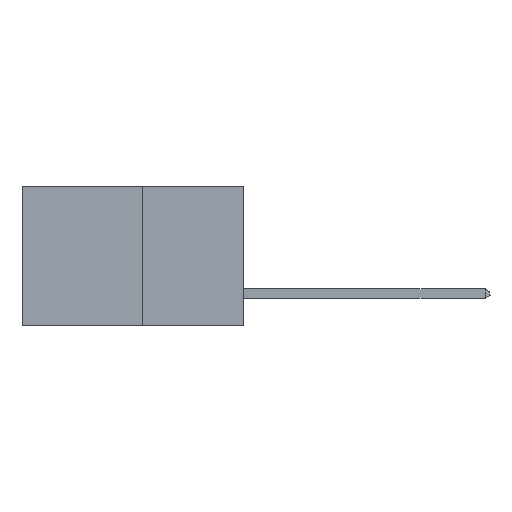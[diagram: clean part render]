
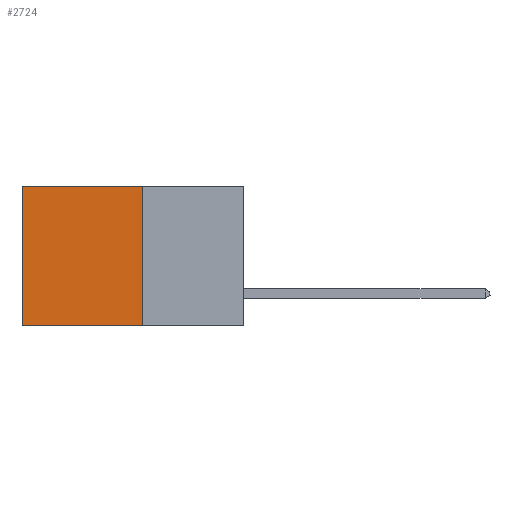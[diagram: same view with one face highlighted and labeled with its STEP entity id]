
A CAD part, left-side view. The second image highlights one B-rep face of the part: STEP entity #2724.
In plain terms, the highlighted planar face has unit normal (-1, 0, 0).
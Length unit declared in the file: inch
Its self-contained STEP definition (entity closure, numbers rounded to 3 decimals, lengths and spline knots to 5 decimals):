
#101 = AXIS2_PLACEMENT_3D ( 'NONE', #4078, #1665, #5378 ) ;
#337 = DIRECTION ( 'NONE',  ( 0., 1., 0. ) ) ;
#406 = DIRECTION ( 'NONE',  ( 0., 0., -1. ) ) ;
#720 = VERTEX_POINT ( 'NONE', #4737 ) ;
#1048 = CARTESIAN_POINT ( 'NONE',  ( 0.277, 0.27, -0.37 ) ) ;
#1312 = VECTOR ( 'NONE', #9740, 39.37008 ) ;
#1665 = DIRECTION ( 'NONE',  ( 1., 0., 0. ) ) ;
#2157 = EDGE_CURVE ( 'NONE', #720, #2287, #6158, .T. ) ;
#2287 = VERTEX_POINT ( 'NONE', #7192 ) ;
#2482 = ORIENTED_EDGE ( 'NONE', *, *, #2157, .T. ) ;
#2593 = ORIENTED_EDGE ( 'NONE', *, *, #8492, .F. ) ;
#2691 = ORIENTED_EDGE ( 'NONE', *, *, #5030, .F. ) ;
#2724 = ADVANCED_FACE ( 'NONE', ( #8863 ), #6753, .F. ) ;
#2806 = ORIENTED_EDGE ( 'NONE', *, *, #6980, .T. ) ;
#3305 = LINE ( 'NONE', #10052, #7297 ) ;
#4046 = DIRECTION ( 'NONE',  ( 0., 1., 0. ) ) ;
#4078 = CARTESIAN_POINT ( 'NONE',  ( 0.277, 0.27, -0.37 ) ) ;
#4116 = LINE ( 'NONE', #1048, #8066 ) ;
#4737 = CARTESIAN_POINT ( 'NONE',  ( 0.277, 0.59, 0. ) ) ;
#5030 = EDGE_CURVE ( 'NONE', #8973, #7279, #4116, .T. ) ;
#5196 = CARTESIAN_POINT ( 'NONE',  ( 0.277, 0.27, 0. ) ) ;
#5378 = DIRECTION ( 'NONE',  ( 0., 0., -1. ) ) ;
#5487 = LINE ( 'NONE', #9449, #9608 ) ;
#6158 = LINE ( 'NONE', #8176, #1312 ) ;
#6753 = PLANE ( 'NONE',  #101 ) ;
#6980 = EDGE_CURVE ( 'NONE', #8973, #720, #5487, .T. ) ;
#7192 = CARTESIAN_POINT ( 'NONE',  ( 0.277, 0.59, -0.37 ) ) ;
#7279 = VERTEX_POINT ( 'NONE', #10397 ) ;
#7297 = VECTOR ( 'NONE', #337, 39.37008 ) ;
#7553 = EDGE_LOOP ( 'NONE', ( #2482, #2593, #2691, #2806 ) ) ;
#8066 = VECTOR ( 'NONE', #406, 39.37008 ) ;
#8176 = CARTESIAN_POINT ( 'NONE',  ( 0.277, 0.59, -0.37 ) ) ;
#8492 = EDGE_CURVE ( 'NONE', #7279, #2287, #3305, .T. ) ;
#8863 = FACE_OUTER_BOUND ( 'NONE', #7553, .T. ) ;
#8973 = VERTEX_POINT ( 'NONE', #5196 ) ;
#9449 = CARTESIAN_POINT ( 'NONE',  ( 0.277, 0.27, 0. ) ) ;
#9608 = VECTOR ( 'NONE', #4046, 39.37008 ) ;
#9740 = DIRECTION ( 'NONE',  ( 0., 0., -1. ) ) ;
#10052 = CARTESIAN_POINT ( 'NONE',  ( 0.277, 0.27, -0.37 ) ) ;
#10397 = CARTESIAN_POINT ( 'NONE',  ( 0.277, 0.27, -0.37 ) ) ;
